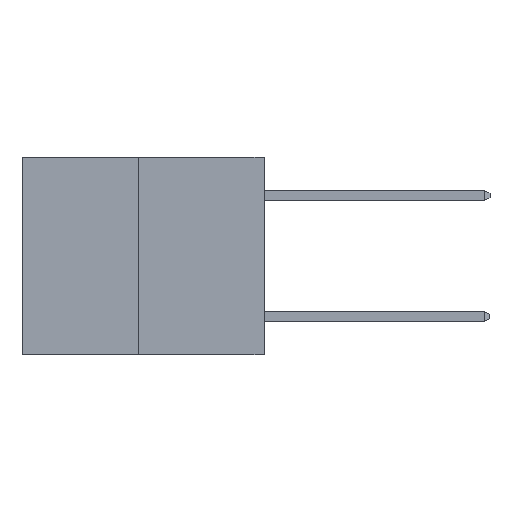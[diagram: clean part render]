
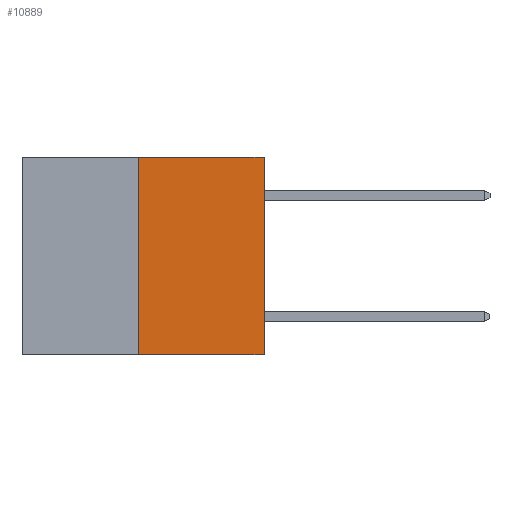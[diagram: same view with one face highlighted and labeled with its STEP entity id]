
A CAD part, left-side view. The second image highlights one B-rep face of the part: STEP entity #10889.
In plain terms, the highlighted planar face has unit normal (-1, 0, 0).
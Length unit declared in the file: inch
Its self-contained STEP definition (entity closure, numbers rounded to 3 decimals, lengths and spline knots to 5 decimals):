
#949 = ORIENTED_EDGE ( 'NONE', *, *, #6550, .F. ) ;
#1168 = FACE_OUTER_BOUND ( 'NONE', #13162, .T. ) ;
#3075 = VERTEX_POINT ( 'NONE', #4797 ) ;
#3107 = LINE ( 'NONE', #13167, #7019 ) ;
#3971 = VERTEX_POINT ( 'NONE', #11441 ) ;
#4797 = CARTESIAN_POINT ( 'NONE',  ( 0., 0.312, 0. ) ) ;
#5328 = VERTEX_POINT ( 'NONE', #21145 ) ;
#5390 = VERTEX_POINT ( 'NONE', #9939 ) ;
#5440 = CARTESIAN_POINT ( 'NONE',  ( 0., 0.6, -0.49 ) ) ;
#6051 = VECTOR ( 'NONE', #12386, 39.37008 ) ;
#6125 = ORIENTED_EDGE ( 'NONE', *, *, #13605, .T. ) ;
#6550 = EDGE_CURVE ( 'NONE', #3075, #5328, #10453, .T. ) ;
#6883 = DIRECTION ( 'NONE',  ( 0., 0., -1. ) ) ;
#7019 = VECTOR ( 'NONE', #18037, 39.37008 ) ;
#7080 = ORIENTED_EDGE ( 'NONE', *, *, #9966, .T. ) ;
#8283 = LINE ( 'NONE', #17883, #16646 ) ;
#8300 = EDGE_CURVE ( 'NONE', #5390, #3075, #3107, .T. ) ;
#8348 = DIRECTION ( 'NONE',  ( 1., 0., 0. ) ) ;
#9541 = ORIENTED_EDGE ( 'NONE', *, *, #8300, .F. ) ;
#9939 = CARTESIAN_POINT ( 'NONE',  ( 0., 0.312, -0.49 ) ) ;
#9966 = EDGE_CURVE ( 'NONE', #3971, #5328, #8283, .T. ) ;
#10365 = DIRECTION ( 'NONE',  ( 0., -1., 0. ) ) ;
#10453 = LINE ( 'NONE', #10769, #6051 ) ;
#10769 = CARTESIAN_POINT ( 'NONE',  ( 0., 0.6, 0. ) ) ;
#10889 = ADVANCED_FACE ( 'NONE', ( #1168 ), #19550, .F. ) ;
#11441 = CARTESIAN_POINT ( 'NONE',  ( 0., 0., -0.49 ) ) ;
#12386 = DIRECTION ( 'NONE',  ( 0., -1., 0. ) ) ;
#13162 = EDGE_LOOP ( 'NONE', ( #9541, #6125, #7080, #949 ) ) ;
#13167 = CARTESIAN_POINT ( 'NONE',  ( 0., 0.312, -0.49 ) ) ;
#13605 = EDGE_CURVE ( 'NONE', #5390, #3971, #17529, .T. ) ;
#14084 = AXIS2_PLACEMENT_3D ( 'NONE', #16956, #8348, #6883 ) ;
#16646 = VECTOR ( 'NONE', #19697, 39.37008 ) ;
#16956 = CARTESIAN_POINT ( 'NONE',  ( 0., 0.6, 0. ) ) ;
#17529 = LINE ( 'NONE', #5440, #20861 ) ;
#17883 = CARTESIAN_POINT ( 'NONE',  ( 0., 0., 0. ) ) ;
#18037 = DIRECTION ( 'NONE',  ( 0., 0., 1. ) ) ;
#19550 = PLANE ( 'NONE',  #14084 ) ;
#19697 = DIRECTION ( 'NONE',  ( 0., 0., 1. ) ) ;
#20861 = VECTOR ( 'NONE', #10365, 39.37008 ) ;
#21145 = CARTESIAN_POINT ( 'NONE',  ( 0., 0., 0. ) ) ;
